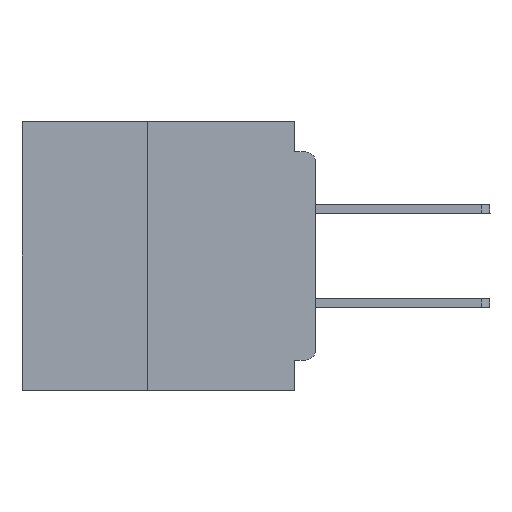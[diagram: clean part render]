
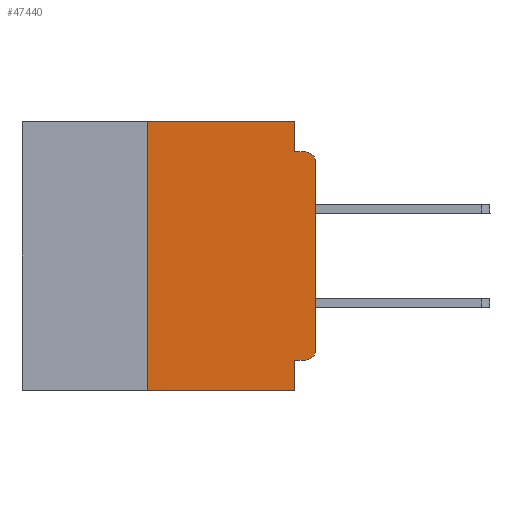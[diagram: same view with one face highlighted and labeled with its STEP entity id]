
A CAD part, left-side view. The second image highlights one B-rep face of the part: STEP entity #47440.
In plain terms, the highlighted planar face has unit normal (-1, 0, 0).
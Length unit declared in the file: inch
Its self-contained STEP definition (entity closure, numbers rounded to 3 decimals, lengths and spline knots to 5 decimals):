
#14 = ORIENTED_EDGE ( 'NONE', *, *, #34834, .F. ) ;
#101 = DIRECTION ( 'NONE',  ( 0., 0., 1. ) ) ;
#183 = CARTESIAN_POINT ( 'NONE',  ( 0., 0.25, 0. ) ) ;
#2913 = VERTEX_POINT ( 'NONE', #64452 ) ;
#3837 = EDGE_CURVE ( 'NONE', #42001, #19516, #59167, .T. ) ;
#5725 = CARTESIAN_POINT ( 'NONE',  ( 0., 0.25, -0.4 ) ) ;
#6126 = DIRECTION ( 'NONE',  ( 0., -1., 0. ) ) ;
#6911 = ORIENTED_EDGE ( 'NONE', *, *, #29504, .F. ) ;
#6948 = DIRECTION ( 'NONE',  ( 0., 0., -1. ) ) ;
#7384 = VECTOR ( 'NONE', #15098, 39.37008 ) ;
#7806 = LINE ( 'NONE', #36773, #62093 ) ;
#7885 = VERTEX_POINT ( 'NONE', #5725 ) ;
#8408 = CARTESIAN_POINT ( 'NONE',  ( 0., 0., -0.045 ) ) ;
#8990 = LINE ( 'NONE', #40549, #7384 ) ;
#9858 = CARTESIAN_POINT ( 'NONE',  ( 0., 0.015, -0.06 ) ) ;
#10254 = LINE ( 'NONE', #54453, #37463 ) ;
#11910 = EDGE_CURVE ( 'NONE', #7885, #35060, #8990, .T. ) ;
#13097 = EDGE_CURVE ( 'NONE', #2913, #50543, #57552, .T. ) ;
#13569 = CARTESIAN_POINT ( 'NONE',  ( 0., 0.031, -0.045 ) ) ;
#13590 = CARTESIAN_POINT ( 'NONE',  ( 0., 0.031, 0. ) ) ;
#13752 = CIRCLE ( 'NONE', #14572, 0.015 ) ;
#14572 = AXIS2_PLACEMENT_3D ( 'NONE', #9858, #45608, #15043 ) ;
#14747 = DIRECTION ( 'NONE',  ( -1., 0., 0. ) ) ;
#15043 = DIRECTION ( 'NONE',  ( 0., 0., -1. ) ) ;
#15098 = DIRECTION ( 'NONE',  ( 0., 0., 1. ) ) ;
#15502 = CARTESIAN_POINT ( 'NONE',  ( 0., 0., 0. ) ) ;
#17053 = CARTESIAN_POINT ( 'NONE',  ( 0., 0.437, 0. ) ) ;
#18705 = VECTOR ( 'NONE', #63302, 39.37008 ) ;
#19516 = VERTEX_POINT ( 'NONE', #26797 ) ;
#19563 = VECTOR ( 'NONE', #27519, 39.37008 ) ;
#19740 = VECTOR ( 'NONE', #28980, 39.37008 ) ;
#20068 = VECTOR ( 'NONE', #51019, 39.37008 ) ;
#20461 = CARTESIAN_POINT ( 'NONE',  ( 0., 0.031, -0.4 ) ) ;
#21680 = VECTOR ( 'NONE', #101, 39.37008 ) ;
#22224 = EDGE_CURVE ( 'NONE', #51763, #32614, #13752, .T. ) ;
#23906 = DIRECTION ( 'NONE',  ( 0., 0., -1. ) ) ;
#24348 = EDGE_CURVE ( 'NONE', #2913, #42001, #57809, .T. ) ;
#24754 = ORIENTED_EDGE ( 'NONE', *, *, #13097, .T. ) ;
#26702 = EDGE_CURVE ( 'NONE', #50543, #51763, #48766, .T. ) ;
#26797 = CARTESIAN_POINT ( 'NONE',  ( 0., 0.031, -0.4 ) ) ;
#27076 = AXIS2_PLACEMENT_3D ( 'NONE', #17053, #37585, #6948 ) ;
#27519 = DIRECTION ( 'NONE',  ( 0., -1., 0. ) ) ;
#28980 = DIRECTION ( 'NONE',  ( 0., -1., 0. ) ) ;
#29504 = EDGE_CURVE ( 'NONE', #35060, #63945, #46717, .T. ) ;
#29651 = ORIENTED_EDGE ( 'NONE', *, *, #64304, .T. ) ;
#32442 = PLANE ( 'NONE',  #27076 ) ;
#32614 = VERTEX_POINT ( 'NONE', #36529 ) ;
#33299 = LINE ( 'NONE', #8408, #19740 ) ;
#34834 = EDGE_CURVE ( 'NONE', #59182, #32614, #33299, .T. ) ;
#35060 = VERTEX_POINT ( 'NONE', #183 ) ;
#36529 = CARTESIAN_POINT ( 'NONE',  ( 0., 0.015, -0.045 ) ) ;
#36773 = CARTESIAN_POINT ( 'NONE',  ( 0., 0.437, -0.4 ) ) ;
#37463 = VECTOR ( 'NONE', #23906, 39.37008 ) ;
#37585 = DIRECTION ( 'NONE',  ( 1., 0., 0. ) ) ;
#39352 = ORIENTED_EDGE ( 'NONE', *, *, #24348, .F. ) ;
#39482 = CARTESIAN_POINT ( 'NONE',  ( 0., 0., -0.34 ) ) ;
#40383 = EDGE_CURVE ( 'NONE', #63945, #59182, #10254, .T. ) ;
#40549 = CARTESIAN_POINT ( 'NONE',  ( 0., 0.25, -0.4 ) ) ;
#41348 = EDGE_LOOP ( 'NONE', ( #47737, #53613, #14, #62436, #6911, #45043, #29651, #52144, #39352, #24754 ) ) ;
#42001 = VERTEX_POINT ( 'NONE', #56716 ) ;
#45043 = ORIENTED_EDGE ( 'NONE', *, *, #11910, .F. ) ;
#45323 = CARTESIAN_POINT ( 'NONE',  ( 0., 0.015, -0.34 ) ) ;
#45608 = DIRECTION ( 'NONE',  ( -1., 0., 0. ) ) ;
#46717 = LINE ( 'NONE', #63121, #19563 ) ;
#47440 = ADVANCED_FACE ( 'NONE', ( #54856 ), #32442, .F. ) ;
#47737 = ORIENTED_EDGE ( 'NONE', *, *, #26702, .T. ) ;
#48766 = LINE ( 'NONE', #15502, #21680 ) ;
#48883 = CARTESIAN_POINT ( 'NONE',  ( 0., 0., -0.06 ) ) ;
#50399 = DIRECTION ( 'NONE',  ( 0., 0., -1. ) ) ;
#50543 = VERTEX_POINT ( 'NONE', #39482 ) ;
#51019 = DIRECTION ( 'NONE',  ( 0., 0., -1. ) ) ;
#51763 = VERTEX_POINT ( 'NONE', #48883 ) ;
#52144 = ORIENTED_EDGE ( 'NONE', *, *, #3837, .F. ) ;
#53613 = ORIENTED_EDGE ( 'NONE', *, *, #22224, .T. ) ;
#54453 = CARTESIAN_POINT ( 'NONE',  ( 0., 0.031, 0. ) ) ;
#54856 = FACE_OUTER_BOUND ( 'NONE', #41348, .T. ) ;
#56716 = CARTESIAN_POINT ( 'NONE',  ( 0., 0.031, -0.355 ) ) ;
#57552 = CIRCLE ( 'NONE', #58632, 0.015 ) ;
#57809 = LINE ( 'NONE', #58215, #18705 ) ;
#58215 = CARTESIAN_POINT ( 'NONE',  ( 0., 0., -0.355 ) ) ;
#58632 = AXIS2_PLACEMENT_3D ( 'NONE', #45323, #14747, #50399 ) ;
#59167 = LINE ( 'NONE', #20461, #20068 ) ;
#59182 = VERTEX_POINT ( 'NONE', #13569 ) ;
#62093 = VECTOR ( 'NONE', #6126, 39.37008 ) ;
#62436 = ORIENTED_EDGE ( 'NONE', *, *, #40383, .F. ) ;
#63121 = CARTESIAN_POINT ( 'NONE',  ( 0., 0.437, 0. ) ) ;
#63302 = DIRECTION ( 'NONE',  ( 0., 1., 0. ) ) ;
#63945 = VERTEX_POINT ( 'NONE', #13590 ) ;
#64304 = EDGE_CURVE ( 'NONE', #7885, #19516, #7806, .T. ) ;
#64452 = CARTESIAN_POINT ( 'NONE',  ( 0., 0.015, -0.355 ) ) ;
